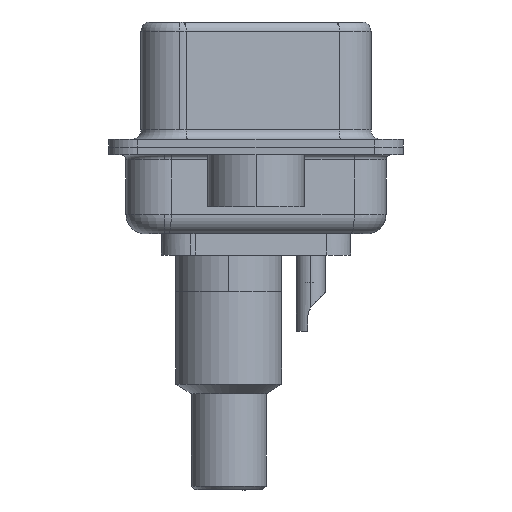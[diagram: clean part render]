
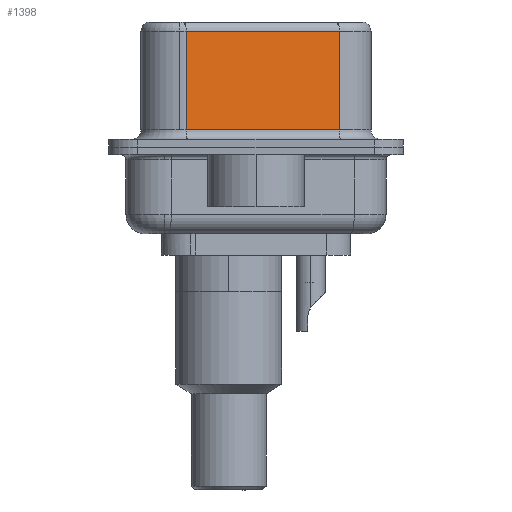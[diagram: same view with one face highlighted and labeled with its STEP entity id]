
A CAD part, left-side view. The second image highlights one B-rep face of the part: STEP entity #1398.
In plain terms, the highlighted planar face has unit normal (-0.985, -0.174, 0).
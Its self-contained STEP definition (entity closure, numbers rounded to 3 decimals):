
#360 = CARTESIAN_POINT ( 'NONE',  ( 5.132, -4.322, 6.02 ) ) ;
#424 = LINE ( 'NONE', #360, #10003 ) ;
#1398 = ADVANCED_FACE ( 'NONE', ( #23910 ), #21136, .F. ) ;
#1768 = ORIENTED_EDGE ( 'NONE', *, *, #3555, .F. ) ;
#1935 = DIRECTION ( 'NONE',  ( 0.174, -0.985, 0. ) ) ;
#2866 = VECTOR ( 'NONE', #10943, 1000. ) ;
#3129 = EDGE_CURVE ( 'NONE', #9777, #13913, #7952, .T. ) ;
#3555 = EDGE_CURVE ( 'NONE', #16678, #9744, #4660, .T. ) ;
#3750 = EDGE_CURVE ( 'NONE', #16678, #9777, #424, .T. ) ;
#4660 = LINE ( 'NONE', #14677, #19355 ) ;
#4722 = EDGE_LOOP ( 'NONE', ( #1768, #17585, #21782, #15979 ) ) ;
#6321 = CARTESIAN_POINT ( 'NONE',  ( 5.132, -4.322, 0.9 ) ) ;
#6935 = DIRECTION ( 'NONE',  ( 0., 0., -1. ) ) ;
#7235 = DIRECTION ( 'NONE',  ( -0.174, 0.985, 0. ) ) ;
#7469 = CARTESIAN_POINT ( 'NONE',  ( 5.132, -4.322, 6.02 ) ) ;
#7952 = LINE ( 'NONE', #23708, #2866 ) ;
#8074 = CARTESIAN_POINT ( 'NONE',  ( 5.132, -4.322, 6.52 ) ) ;
#9744 = VERTEX_POINT ( 'NONE', #17332 ) ;
#9771 = CARTESIAN_POINT ( 'NONE',  ( 3.73, 3.628, 6.02 ) ) ;
#9777 = VERTEX_POINT ( 'NONE', #9771 ) ;
#10003 = VECTOR ( 'NONE', #19577, 1000. ) ;
#10943 = DIRECTION ( 'NONE',  ( 0., 0., -1. ) ) ;
#11919 = EDGE_CURVE ( 'NONE', #13913, #9744, #22494, .T. ) ;
#13913 = VERTEX_POINT ( 'NONE', #18277 ) ;
#14677 = CARTESIAN_POINT ( 'NONE',  ( 5.132, -4.322, 6.52 ) ) ;
#15432 = AXIS2_PLACEMENT_3D ( 'NONE', #8074, #15847, #7235 ) ;
#15847 = DIRECTION ( 'NONE',  ( 0.985, 0.174, 0. ) ) ;
#15979 = ORIENTED_EDGE ( 'NONE', *, *, #11919, .T. ) ;
#16678 = VERTEX_POINT ( 'NONE', #7469 ) ;
#17332 = CARTESIAN_POINT ( 'NONE',  ( 5.132, -4.322, 0.9 ) ) ;
#17585 = ORIENTED_EDGE ( 'NONE', *, *, #3750, .T. ) ;
#18277 = CARTESIAN_POINT ( 'NONE',  ( 3.73, 3.628, 0.9 ) ) ;
#19355 = VECTOR ( 'NONE', #6935, 1000. ) ;
#19577 = DIRECTION ( 'NONE',  ( -0.174, 0.985, 0. ) ) ;
#21136 = PLANE ( 'NONE',  #15432 ) ;
#21782 = ORIENTED_EDGE ( 'NONE', *, *, #3129, .T. ) ;
#21906 = VECTOR ( 'NONE', #1935, 1000. ) ;
#22494 = LINE ( 'NONE', #6321, #21906 ) ;
#23708 = CARTESIAN_POINT ( 'NONE',  ( 3.73, 3.628, 6.52 ) ) ;
#23910 = FACE_OUTER_BOUND ( 'NONE', #4722, .T. ) ;
